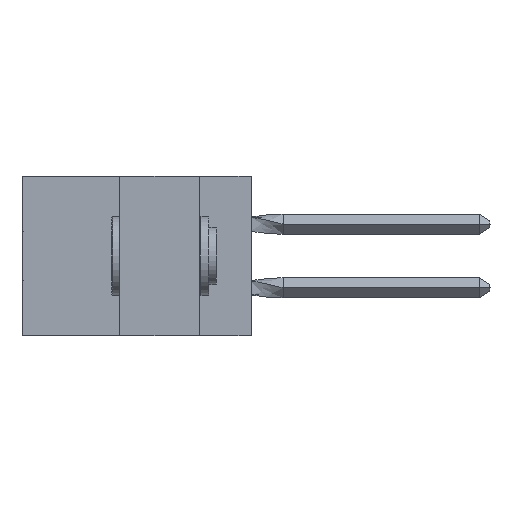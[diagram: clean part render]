
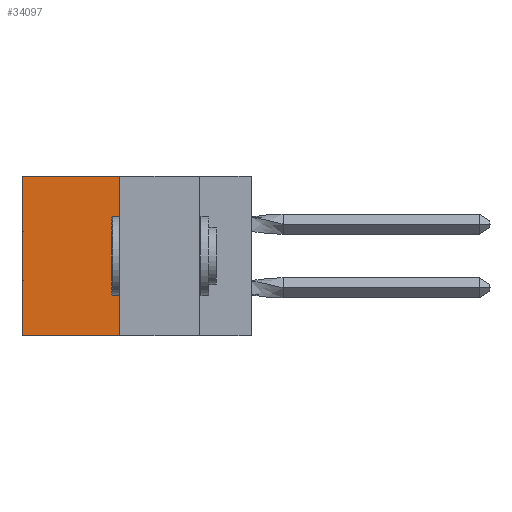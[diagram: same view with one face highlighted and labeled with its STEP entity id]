
A CAD part, left-side view. The second image highlights one B-rep face of the part: STEP entity #34097.
In plain terms, the highlighted planar face has unit normal (-1, 0, 0).
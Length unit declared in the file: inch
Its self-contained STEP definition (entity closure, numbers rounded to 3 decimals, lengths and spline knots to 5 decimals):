
#238 = VECTOR ( 'NONE', #20917, 39.37008 ) ;
#1367 = CARTESIAN_POINT ( 'NONE',  ( 0.305, 0.72, 0. ) ) ;
#2988 = CARTESIAN_POINT ( 'NONE',  ( 0.305, 0.413, -0.5 ) ) ;
#4956 = ORIENTED_EDGE ( 'NONE', *, *, #27400, .F. ) ;
#5301 = CARTESIAN_POINT ( 'NONE',  ( 0.305, 0.413, 0. ) ) ;
#6625 = ORIENTED_EDGE ( 'NONE', *, *, #37460, .T. ) ;
#7692 = LINE ( 'NONE', #27577, #238 ) ;
#8741 = EDGE_LOOP ( 'NONE', ( #6625, #32929, #4956, #47196 ) ) ;
#9207 = LINE ( 'NONE', #15387, #19464 ) ;
#10316 = DIRECTION ( 'NONE',  ( 1., 0., 0. ) ) ;
#10632 = DIRECTION ( 'NONE',  ( 0., 0., -1. ) ) ;
#12444 = LINE ( 'NONE', #13603, #30683 ) ;
#13603 = CARTESIAN_POINT ( 'NONE',  ( 0.305, 0.413, -0.5 ) ) ;
#14246 = VECTOR ( 'NONE', #39243, 39.37008 ) ;
#14802 = EDGE_CURVE ( 'NONE', #22006, #28244, #12444, .T. ) ;
#15387 = CARTESIAN_POINT ( 'NONE',  ( 0.305, 0.413, -0.5 ) ) ;
#19464 = VECTOR ( 'NONE', #40960, 39.37008 ) ;
#20917 = DIRECTION ( 'NONE',  ( 0., 0., -1. ) ) ;
#21440 = VERTEX_POINT ( 'NONE', #5301 ) ;
#22006 = VERTEX_POINT ( 'NONE', #26597 ) ;
#22843 = LINE ( 'NONE', #28025, #14246 ) ;
#24424 = AXIS2_PLACEMENT_3D ( 'NONE', #2988, #10316, #10632 ) ;
#24816 = PLANE ( 'NONE',  #24424 ) ;
#25494 = CARTESIAN_POINT ( 'NONE',  ( 0.305, 0.72, -0.5 ) ) ;
#26597 = CARTESIAN_POINT ( 'NONE',  ( 0.305, 0.413, -0.5 ) ) ;
#27400 = EDGE_CURVE ( 'NONE', #21440, #22006, #9207, .T. ) ;
#27577 = CARTESIAN_POINT ( 'NONE',  ( 0.305, 0.72, -0.5 ) ) ;
#28025 = CARTESIAN_POINT ( 'NONE',  ( 0.305, 0.413, 0. ) ) ;
#28244 = VERTEX_POINT ( 'NONE', #25494 ) ;
#28381 = VERTEX_POINT ( 'NONE', #1367 ) ;
#30683 = VECTOR ( 'NONE', #44678, 39.37008 ) ;
#32238 = EDGE_CURVE ( 'NONE', #21440, #28381, #22843, .T. ) ;
#32929 = ORIENTED_EDGE ( 'NONE', *, *, #14802, .F. ) ;
#34097 = ADVANCED_FACE ( 'NONE', ( #43765 ), #24816, .F. ) ;
#37460 = EDGE_CURVE ( 'NONE', #28381, #28244, #7692, .T. ) ;
#39243 = DIRECTION ( 'NONE',  ( 0., 1., 0. ) ) ;
#40960 = DIRECTION ( 'NONE',  ( 0., 0., -1. ) ) ;
#43765 = FACE_OUTER_BOUND ( 'NONE', #8741, .T. ) ;
#44678 = DIRECTION ( 'NONE',  ( 0., 1., 0. ) ) ;
#47196 = ORIENTED_EDGE ( 'NONE', *, *, #32238, .T. ) ;
